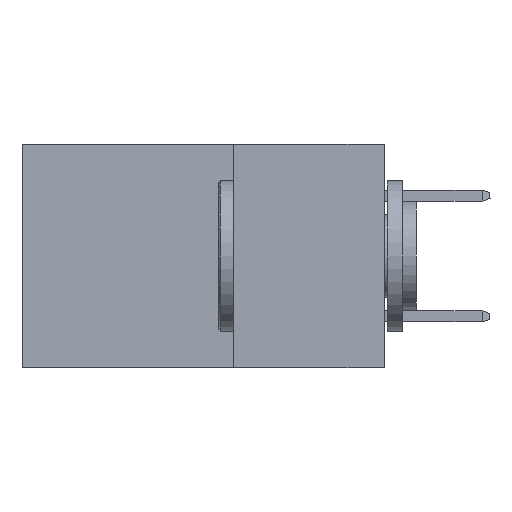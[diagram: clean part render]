
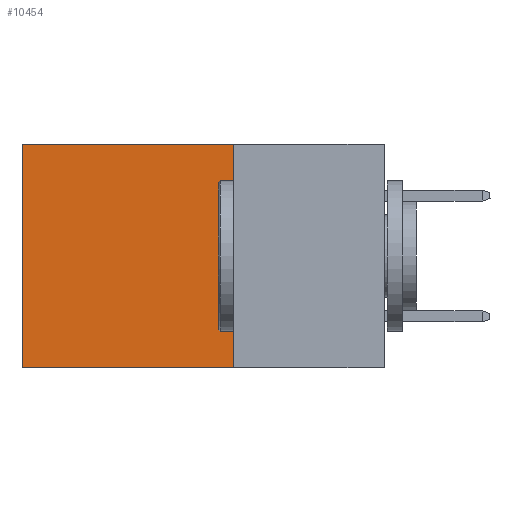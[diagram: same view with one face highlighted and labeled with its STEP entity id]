
A CAD part, left-side view. The second image highlights one B-rep face of the part: STEP entity #10454.
In plain terms, the highlighted planar face has unit normal (-1, 0, 0).
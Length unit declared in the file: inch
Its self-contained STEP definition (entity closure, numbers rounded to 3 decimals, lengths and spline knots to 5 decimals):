
#182 = EDGE_CURVE ( 'NONE', #3043, #6849, #14123, .T. ) ;
#1407 = DIRECTION ( 'NONE',  ( 0., 1., 0. ) ) ;
#1448 = DIRECTION ( 'NONE',  ( 1., 0., 0. ) ) ;
#2550 = VERTEX_POINT ( 'NONE', #4183 ) ;
#3043 = VERTEX_POINT ( 'NONE', #21644 ) ;
#3380 = VERTEX_POINT ( 'NONE', #17270 ) ;
#4183 = CARTESIAN_POINT ( 'NONE',  ( 0.298, 0.25, 0. ) ) ;
#4638 = EDGE_LOOP ( 'NONE', ( #11199, #16655, #11846, #15687 ) ) ;
#4860 = DIRECTION ( 'NONE',  ( 0., 0., -1. ) ) ;
#4947 = CARTESIAN_POINT ( 'NONE',  ( 0.298, 0.6, 0. ) ) ;
#5486 = EDGE_CURVE ( 'NONE', #2550, #3043, #14993, .T. ) ;
#5616 = VECTOR ( 'NONE', #1407, 39.37008 ) ;
#6849 = VERTEX_POINT ( 'NONE', #17579 ) ;
#8316 = DIRECTION ( 'NONE',  ( 0., 0., -1. ) ) ;
#8710 = CARTESIAN_POINT ( 'NONE',  ( 0.298, 0.25, 0. ) ) ;
#10069 = CARTESIAN_POINT ( 'NONE',  ( 0.298, 0.25, 0. ) ) ;
#10454 = ADVANCED_FACE ( 'NONE', ( #16846 ), #12258, .F. ) ;
#11199 = ORIENTED_EDGE ( 'NONE', *, *, #14271, .T. ) ;
#11527 = DIRECTION ( 'NONE',  ( 0., 1., 0. ) ) ;
#11659 = CARTESIAN_POINT ( 'NONE',  ( 0.298, 0.25, -0.37 ) ) ;
#11846 = ORIENTED_EDGE ( 'NONE', *, *, #5486, .F. ) ;
#12258 = PLANE ( 'NONE',  #14289 ) ;
#14054 = DIRECTION ( 'NONE',  ( 0., 0., -1. ) ) ;
#14123 = LINE ( 'NONE', #11659, #19237 ) ;
#14271 = EDGE_CURVE ( 'NONE', #3380, #6849, #17012, .T. ) ;
#14289 = AXIS2_PLACEMENT_3D ( 'NONE', #8710, #1448, #14054 ) ;
#14993 = LINE ( 'NONE', #10069, #19564 ) ;
#15073 = LINE ( 'NONE', #22575, #5616 ) ;
#15687 = ORIENTED_EDGE ( 'NONE', *, *, #19910, .T. ) ;
#16655 = ORIENTED_EDGE ( 'NONE', *, *, #182, .F. ) ;
#16846 = FACE_OUTER_BOUND ( 'NONE', #4638, .T. ) ;
#17012 = LINE ( 'NONE', #4947, #17546 ) ;
#17270 = CARTESIAN_POINT ( 'NONE',  ( 0.298, 0.6, 0. ) ) ;
#17546 = VECTOR ( 'NONE', #4860, 39.37008 ) ;
#17579 = CARTESIAN_POINT ( 'NONE',  ( 0.298, 0.6, -0.37 ) ) ;
#19237 = VECTOR ( 'NONE', #11527, 39.37008 ) ;
#19564 = VECTOR ( 'NONE', #8316, 39.37008 ) ;
#19910 = EDGE_CURVE ( 'NONE', #2550, #3380, #15073, .T. ) ;
#21644 = CARTESIAN_POINT ( 'NONE',  ( 0.298, 0.25, -0.37 ) ) ;
#22575 = CARTESIAN_POINT ( 'NONE',  ( 0.298, 0.25, 0. ) ) ;
